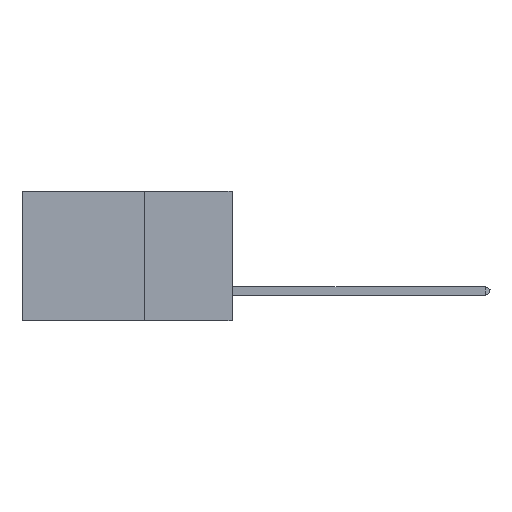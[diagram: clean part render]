
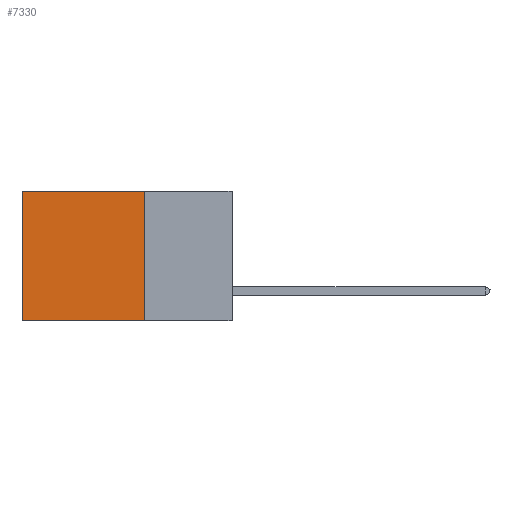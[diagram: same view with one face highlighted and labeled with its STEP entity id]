
A CAD part, left-side view. The second image highlights one B-rep face of the part: STEP entity #7330.
In plain terms, the highlighted planar face has unit normal (-1, 0, 0).
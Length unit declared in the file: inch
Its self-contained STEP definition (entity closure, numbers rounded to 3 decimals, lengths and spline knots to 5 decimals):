
#274 = CARTESIAN_POINT ( 'NONE',  ( 0.2875, 0.25, -0.37 ) ) ;
#990 = EDGE_CURVE ( 'NONE', #11717, #26625, #1068, .T. ) ;
#1068 = LINE ( 'NONE', #9052, #23083 ) ;
#3690 = DIRECTION ( 'NONE',  ( 1., 0., 0. ) ) ;
#7330 = ADVANCED_FACE ( 'NONE', ( #28280 ), #38380, .F. ) ;
#9052 = CARTESIAN_POINT ( 'NONE',  ( 0.2875, 0.6, 0. ) ) ;
#10372 = ORIENTED_EDGE ( 'NONE', *, *, #990, .T. ) ;
#11717 = VERTEX_POINT ( 'NONE', #47021 ) ;
#14009 = VECTOR ( 'NONE', #15624, 39.37008 ) ;
#14807 = VERTEX_POINT ( 'NONE', #36553 ) ;
#15024 = DIRECTION ( 'NONE',  ( 0., 0., -1. ) ) ;
#15624 = DIRECTION ( 'NONE',  ( 0., 1., 0. ) ) ;
#17832 = VECTOR ( 'NONE', #47468, 39.37008 ) ;
#18412 = EDGE_LOOP ( 'NONE', ( #10372, #47337, #46776, #49030 ) ) ;
#18814 = VERTEX_POINT ( 'NONE', #40312 ) ;
#23083 = VECTOR ( 'NONE', #28228, 39.37008 ) ;
#25343 = LINE ( 'NONE', #30500, #14009 ) ;
#25456 = LINE ( 'NONE', #274, #36201 ) ;
#26625 = VERTEX_POINT ( 'NONE', #31500 ) ;
#26918 = DIRECTION ( 'NONE',  ( 0., 1., 0. ) ) ;
#28228 = DIRECTION ( 'NONE',  ( 0., 0., -1. ) ) ;
#28280 = FACE_OUTER_BOUND ( 'NONE', #18412, .T. ) ;
#30500 = CARTESIAN_POINT ( 'NONE',  ( 0.2875, 0.25, 0. ) ) ;
#31500 = CARTESIAN_POINT ( 'NONE',  ( 0.2875, 0.6, -0.37 ) ) ;
#36201 = VECTOR ( 'NONE', #26918, 39.37008 ) ;
#36553 = CARTESIAN_POINT ( 'NONE',  ( 0.2875, 0.25, -0.37 ) ) ;
#37686 = EDGE_CURVE ( 'NONE', #14807, #26625, #25456, .T. ) ;
#37715 = CARTESIAN_POINT ( 'NONE',  ( 0.2875, 0.25, 0. ) ) ;
#38380 = PLANE ( 'NONE',  #38920 ) ;
#38920 = AXIS2_PLACEMENT_3D ( 'NONE', #37715, #3690, #15024 ) ;
#39664 = CARTESIAN_POINT ( 'NONE',  ( 0.2875, 0.25, 0. ) ) ;
#40312 = CARTESIAN_POINT ( 'NONE',  ( 0.2875, 0.25, 0. ) ) ;
#41938 = EDGE_CURVE ( 'NONE', #18814, #14807, #43506, .T. ) ;
#43506 = LINE ( 'NONE', #39664, #17832 ) ;
#46776 = ORIENTED_EDGE ( 'NONE', *, *, #41938, .F. ) ;
#47021 = CARTESIAN_POINT ( 'NONE',  ( 0.2875, 0.6, 0. ) ) ;
#47337 = ORIENTED_EDGE ( 'NONE', *, *, #37686, .F. ) ;
#47468 = DIRECTION ( 'NONE',  ( 0., 0., -1. ) ) ;
#48370 = EDGE_CURVE ( 'NONE', #18814, #11717, #25343, .T. ) ;
#49030 = ORIENTED_EDGE ( 'NONE', *, *, #48370, .T. ) ;
